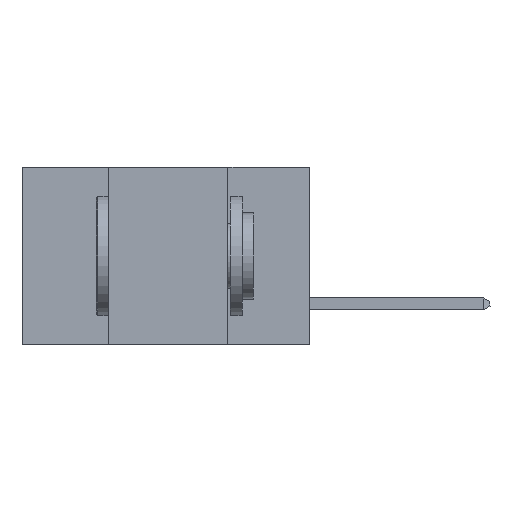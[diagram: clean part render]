
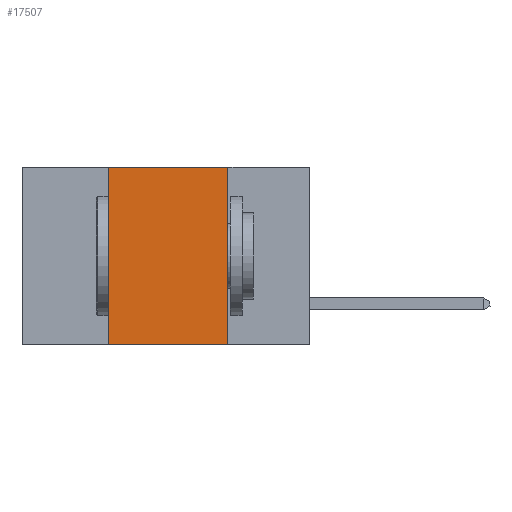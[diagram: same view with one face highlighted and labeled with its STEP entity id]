
A CAD part, left-side view. The second image highlights one B-rep face of the part: STEP entity #17507.
In plain terms, the highlighted planar face has unit normal (-1, 0, 0).
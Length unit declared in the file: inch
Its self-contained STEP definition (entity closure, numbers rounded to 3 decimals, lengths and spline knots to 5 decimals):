
#2141 = CARTESIAN_POINT ( 'NONE',  ( 0., 0.42, 0. ) ) ;
#2579 = ORIENTED_EDGE ( 'NONE', *, *, #3441, .F. ) ;
#3064 = FACE_OUTER_BOUND ( 'NONE', #9369, .T. ) ;
#3162 = VECTOR ( 'NONE', #3401, 39.37008 ) ;
#3335 = EDGE_CURVE ( 'NONE', #12900, #18729, #5488, .T. ) ;
#3350 = DIRECTION ( 'NONE',  ( 0., 0., -1. ) ) ;
#3401 = DIRECTION ( 'NONE',  ( 0., 0., -1. ) ) ;
#3441 = EDGE_CURVE ( 'NONE', #13654, #18729, #14731, .T. ) ;
#4324 = CARTESIAN_POINT ( 'NONE',  ( 0., 0.17, 0. ) ) ;
#4428 = EDGE_CURVE ( 'NONE', #12900, #5258, #6381, .T. ) ;
#5018 = VECTOR ( 'NONE', #11985, 39.37008 ) ;
#5258 = VERTEX_POINT ( 'NONE', #2141 ) ;
#5488 = LINE ( 'NONE', #12092, #5018 ) ;
#6381 = LINE ( 'NONE', #17150, #17380 ) ;
#6446 = CARTESIAN_POINT ( 'NONE',  ( 0., 0.6, 0. ) ) ;
#6863 = CARTESIAN_POINT ( 'NONE',  ( 0., 0.42, -0.37 ) ) ;
#9176 = AXIS2_PLACEMENT_3D ( 'NONE', #10720, #12101, #3350 ) ;
#9369 = EDGE_LOOP ( 'NONE', ( #2579, #12392, #12466, #10951 ) ) ;
#9846 = LINE ( 'NONE', #6446, #17832 ) ;
#10720 = CARTESIAN_POINT ( 'NONE',  ( 0., 0.6, 0. ) ) ;
#10951 = ORIENTED_EDGE ( 'NONE', *, *, #3335, .T. ) ;
#11189 = EDGE_CURVE ( 'NONE', #5258, #13654, #9846, .T. ) ;
#11985 = DIRECTION ( 'NONE',  ( 0., -1., 0. ) ) ;
#12092 = CARTESIAN_POINT ( 'NONE',  ( 0., 0.6, -0.37 ) ) ;
#12101 = DIRECTION ( 'NONE',  ( 1., 0., 0. ) ) ;
#12392 = ORIENTED_EDGE ( 'NONE', *, *, #11189, .F. ) ;
#12466 = ORIENTED_EDGE ( 'NONE', *, *, #4428, .F. ) ;
#12900 = VERTEX_POINT ( 'NONE', #6863 ) ;
#13654 = VERTEX_POINT ( 'NONE', #14418 ) ;
#14418 = CARTESIAN_POINT ( 'NONE',  ( 0., 0.17, 0. ) ) ;
#14731 = LINE ( 'NONE', #4324, #3162 ) ;
#15065 = DIRECTION ( 'NONE',  ( 0., -1., 0. ) ) ;
#16311 = PLANE ( 'NONE',  #9176 ) ;
#16957 = DIRECTION ( 'NONE',  ( 0., 0., 1. ) ) ;
#17150 = CARTESIAN_POINT ( 'NONE',  ( 0., 0.42, 0. ) ) ;
#17362 = CARTESIAN_POINT ( 'NONE',  ( 0., 0.17, -0.37 ) ) ;
#17380 = VECTOR ( 'NONE', #16957, 39.37008 ) ;
#17507 = ADVANCED_FACE ( 'NONE', ( #3064 ), #16311, .F. ) ;
#17832 = VECTOR ( 'NONE', #15065, 39.37008 ) ;
#18729 = VERTEX_POINT ( 'NONE', #17362 ) ;
